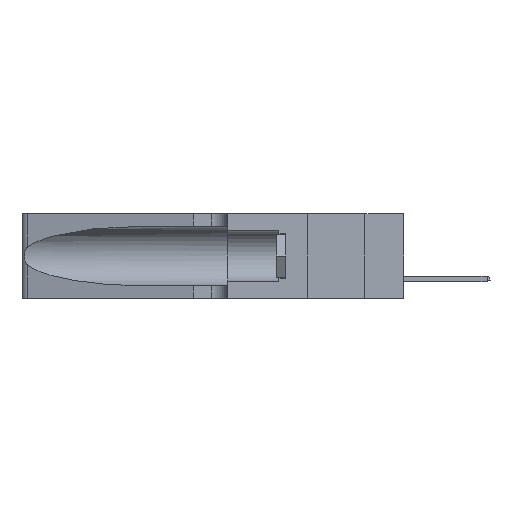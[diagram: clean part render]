
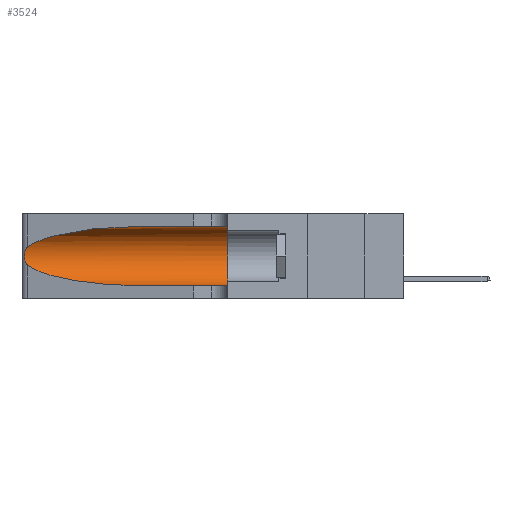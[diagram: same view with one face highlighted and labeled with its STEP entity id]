
A CAD part, left-side view. The second image highlights one B-rep face of the part: STEP entity #3524.
In plain terms, the highlighted cylindrical face has radius 3.308 mm (diameter 6.617 mm), a partial arc.
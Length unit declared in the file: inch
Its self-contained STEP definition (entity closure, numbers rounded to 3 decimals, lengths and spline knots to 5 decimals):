
#104 = CARTESIAN_POINT ( 'NONE',  ( 0.25854, 1.2359, 0.20912 ) ) ;
#889 = ORIENTED_EDGE ( 'NONE', *, *, #5998, .T. ) ;
#1055 = DIRECTION ( 'NONE',  ( 0., -1., 0. ) ) ;
#1140 = DIRECTION ( 'NONE',  ( 0., 0., -1. ) ) ;
#1672 = EDGE_CURVE ( 'NONE', #20056, #23599, #5088, .T. ) ;
#1838 = CARTESIAN_POINT ( 'NONE',  ( 0.25487, 1.22718, 0.14631 ) ) ;
#1962 = ORIENTED_EDGE ( 'NONE', *, *, #12114, .T. ) ;
#2334 = CARTESIAN_POINT ( 'NONE',  ( 0.26017, 1.23833, 0.17102 ) ) ;
#3524 = ADVANCED_FACE ( 'NONE', ( #13933 ), #19889, .F. ) ;
#4202 = ORIENTED_EDGE ( 'NONE', *, *, #7952, .F. ) ;
#4361 = CARTESIAN_POINT ( 'NONE',  ( 0.1305, 1.61858, 0.05475 ) ) ;
#5088 =( BOUNDED_CURVE ( )  B_SPLINE_CURVE ( 3, ( #15417, #10738, #8394, #28832 ),
 .UNSPECIFIED., .F., .T. ) 
 B_SPLINE_CURVE_WITH_KNOTS ( ( 4, 4 ),
 ( 1.5708, 2.84003 ),
 .UNSPECIFIED. ) 
 CURVE ( )  GEOMETRIC_REPRESENTATION_ITEM ( )  RATIONAL_B_SPLINE_CURVE ( ( 1., 0.87, 0.87, 1. ) ) 
 REPRESENTATION_ITEM ( '' )  );
#5998 = EDGE_CURVE ( 'NONE', #9211, #25590, #27363, .T. ) ;
#6939 = CARTESIAN_POINT ( 'NONE',  ( 0.25787, 1.23484, 0.2124 ) ) ;
#7129 = CARTESIAN_POINT ( 'NONE',  ( 0.25487, 1.22718, 0.22369 ) ) ;
#7952 = EDGE_CURVE ( 'NONE', #20056, #9312, #19547, .T. ) ;
#8394 = CARTESIAN_POINT ( 'NONE',  ( 0.2373, 1.15595, 0.28018 ) ) ;
#8589 = CARTESIAN_POINT ( 'NONE',  ( 0.1305, 0.35, 0.05475 ) ) ;
#9211 = VERTEX_POINT ( 'NONE', #10469 ) ;
#9312 = VERTEX_POINT ( 'NONE', #13184 ) ;
#10080 = CARTESIAN_POINT ( 'NONE',  ( 0.25487, 1.22718, 0.22369 ) ) ;
#10469 = CARTESIAN_POINT ( 'NONE',  ( 0.1305, 0.72297, 0.05475 ) ) ;
#10738 = CARTESIAN_POINT ( 'NONE',  ( 0.18966, 0.96281, 0.31525 ) ) ;
#12114 = EDGE_CURVE ( 'NONE', #23599, #17056, #20306, .T. ) ;
#12379 = ORIENTED_EDGE ( 'NONE', *, *, #1672, .T. ) ;
#12606 = DIRECTION ( 'NONE',  ( 0., 0., 1. ) ) ;
#12785 =( BOUNDED_CURVE ( )  B_SPLINE_CURVE ( 3, ( #20525, #25300, #16406, #25209 ),
 .UNSPECIFIED., .F., .T. ) 
 B_SPLINE_CURVE_WITH_KNOTS ( ( 4, 4 ),
 ( 3.44316, 4.71239 ),
 .UNSPECIFIED. ) 
 CURVE ( )  GEOMETRIC_REPRESENTATION_ITEM ( )  RATIONAL_B_SPLINE_CURVE ( ( 1., 0.87, 0.87, 1. ) ) 
 REPRESENTATION_ITEM ( '' )  );
#13184 = CARTESIAN_POINT ( 'NONE',  ( 0.1305, 0.35, 0.31525 ) ) ;
#13858 = CARTESIAN_POINT ( 'NONE',  ( 0.25639, 1.23184, 0.21858 ) ) ;
#13933 = FACE_OUTER_BOUND ( 'NONE', #27046, .T. ) ;
#14512 = CARTESIAN_POINT ( 'NONE',  ( 0.1305, 1.61858, 0.185 ) ) ;
#15417 = CARTESIAN_POINT ( 'NONE',  ( 0.1305, 0.72297, 0.31525 ) ) ;
#15730 = CARTESIAN_POINT ( 'NONE',  ( 0.26075, 1.23896, 0.178 ) ) ;
#16195 = CARTESIAN_POINT ( 'NONE',  ( 0.25789, 1.23486, 0.15765 ) ) ;
#16406 = CARTESIAN_POINT ( 'NONE',  ( 0.18966, 0.96281, 0.05475 ) ) ;
#16600 = DIRECTION ( 'NONE',  ( 0., -1., 0. ) ) ;
#16981 = DIRECTION ( 'NONE',  ( 0., 1., 0. ) ) ;
#17056 = VERTEX_POINT ( 'NONE', #1838 ) ;
#17461 = EDGE_CURVE ( 'NONE', #17056, #9211, #12785, .T. ) ;
#17960 = CARTESIAN_POINT ( 'NONE',  ( 0.25856, 1.23593, 0.16098 ) ) ;
#18457 = CARTESIAN_POINT ( 'NONE',  ( 0.25639, 1.23186, 0.15144 ) ) ;
#18853 = VECTOR ( 'NONE', #16600, 39.37008 ) ;
#19464 = ORIENTED_EDGE ( 'NONE', *, *, #17461, .T. ) ;
#19547 = LINE ( 'NONE', #25786, #18853 ) ;
#19889 = CYLINDRICAL_SURFACE ( 'NONE', #26485, 0.13025 ) ;
#20056 = VERTEX_POINT ( 'NONE', #21815 ) ;
#20155 = ORIENTED_EDGE ( 'NONE', *, *, #28134, .F. ) ;
#20306 = B_SPLINE_CURVE_WITH_KNOTS ( 'NONE', 3,
 ( #7129, #20410, #13858, #6939, #104, #22465, #24708, #15730, #2334, #17960, #16195, #18457, #22844, #20892 ),
 .UNSPECIFIED., .F., .F.,
 ( 4, 2, 2, 2, 2, 2, 4 ),
 ( 0., 0.00027, 0.00053, 0.00107, 0.0016, 0.00187, 0.00214 ),
 .UNSPECIFIED. ) ;
#20410 = CARTESIAN_POINT ( 'NONE',  ( 0.25555, 1.22994, 0.2215 ) ) ;
#20525 = CARTESIAN_POINT ( 'NONE',  ( 0.25487, 1.22718, 0.14631 ) ) ;
#20892 = CARTESIAN_POINT ( 'NONE',  ( 0.25487, 1.22718, 0.14631 ) ) ;
#21386 = CARTESIAN_POINT ( 'NONE',  ( 0.1305, 0.35, 0.185 ) ) ;
#21599 = CIRCLE ( 'NONE', #27594, 0.13025 ) ;
#21815 = CARTESIAN_POINT ( 'NONE',  ( 0.1305, 0.72297, 0.31525 ) ) ;
#22465 = CARTESIAN_POINT ( 'NONE',  ( 0.26018, 1.23835, 0.19895 ) ) ;
#22844 = CARTESIAN_POINT ( 'NONE',  ( 0.25555, 1.22993, 0.14849 ) ) ;
#23599 = VERTEX_POINT ( 'NONE', #10080 ) ;
#24708 = CARTESIAN_POINT ( 'NONE',  ( 0.26075, 1.23896, 0.19203 ) ) ;
#25209 = CARTESIAN_POINT ( 'NONE',  ( 0.1305, 0.72297, 0.05475 ) ) ;
#25259 = VECTOR ( 'NONE', #28606, 39.37008 ) ;
#25300 = CARTESIAN_POINT ( 'NONE',  ( 0.2373, 1.15595, 0.08982 ) ) ;
#25590 = VERTEX_POINT ( 'NONE', #8589 ) ;
#25786 = CARTESIAN_POINT ( 'NONE',  ( 0.1305, 1.61858, 0.31525 ) ) ;
#26485 = AXIS2_PLACEMENT_3D ( 'NONE', #14512, #1055, #1140 ) ;
#27046 = EDGE_LOOP ( 'NONE', ( #12379, #1962, #19464, #889, #20155, #4202 ) ) ;
#27363 = LINE ( 'NONE', #4361, #25259 ) ;
#27594 = AXIS2_PLACEMENT_3D ( 'NONE', #21386, #16981, #12606 ) ;
#28134 = EDGE_CURVE ( 'NONE', #9312, #25590, #21599, .T. ) ;
#28606 = DIRECTION ( 'NONE',  ( 0., -1., 0. ) ) ;
#28832 = CARTESIAN_POINT ( 'NONE',  ( 0.25487, 1.22718, 0.22369 ) ) ;
